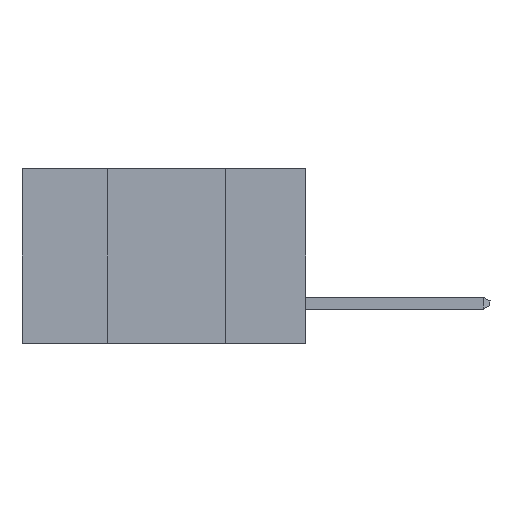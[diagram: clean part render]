
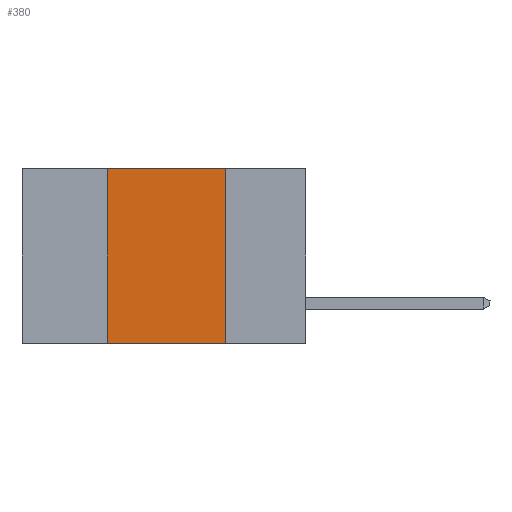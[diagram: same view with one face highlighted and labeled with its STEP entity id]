
A CAD part, left-side view. The second image highlights one B-rep face of the part: STEP entity #380.
In plain terms, the highlighted planar face has unit normal (-1, 0, 0).
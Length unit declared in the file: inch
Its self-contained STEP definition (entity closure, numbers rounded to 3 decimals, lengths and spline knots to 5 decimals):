
#60 = EDGE_LOOP ( 'NONE', ( #5931, #14650, #10827, #14016 ) ) ;
#380 = ADVANCED_FACE ( 'NONE', ( #4554 ), #8325, .F. ) ;
#771 = EDGE_CURVE ( 'NONE', #11678, #6938, #6595, .T. ) ;
#1671 = DIRECTION ( 'NONE',  ( 0., -1., 0. ) ) ;
#2271 = DIRECTION ( 'NONE',  ( 0., -1., 0. ) ) ;
#2495 = EDGE_CURVE ( 'NONE', #8354, #11678, #5177, .T. ) ;
#2605 = CARTESIAN_POINT ( 'NONE',  ( 0., 0.6, 0. ) ) ;
#3304 = LINE ( 'NONE', #3466, #9718 ) ;
#3466 = CARTESIAN_POINT ( 'NONE',  ( 0., 0.42, -0.37 ) ) ;
#4554 = FACE_OUTER_BOUND ( 'NONE', #60, .T. ) ;
#5177 = LINE ( 'NONE', #2605, #11766 ) ;
#5626 = CARTESIAN_POINT ( 'NONE',  ( 0., 0.42, -0.37 ) ) ;
#5931 = ORIENTED_EDGE ( 'NONE', *, *, #771, .F. ) ;
#6094 = LINE ( 'NONE', #8217, #9256 ) ;
#6595 = LINE ( 'NONE', #10203, #14183 ) ;
#6938 = VERTEX_POINT ( 'NONE', #8489 ) ;
#8171 = DIRECTION ( 'NONE',  ( 0., 0., 1. ) ) ;
#8217 = CARTESIAN_POINT ( 'NONE',  ( 0., 0.6, -0.37 ) ) ;
#8325 = PLANE ( 'NONE',  #10686 ) ;
#8354 = VERTEX_POINT ( 'NONE', #15215 ) ;
#8489 = CARTESIAN_POINT ( 'NONE',  ( 0., 0.17, -0.37 ) ) ;
#9256 = VECTOR ( 'NONE', #2271, 39.37008 ) ;
#9366 = CARTESIAN_POINT ( 'NONE',  ( 0., 0.6, 0. ) ) ;
#9718 = VECTOR ( 'NONE', #8171, 39.37008 ) ;
#10203 = CARTESIAN_POINT ( 'NONE',  ( 0., 0.17, -0.37 ) ) ;
#10682 = DIRECTION ( 'NONE',  ( 0., 0., -1. ) ) ;
#10686 = AXIS2_PLACEMENT_3D ( 'NONE', #9366, #12861, #10682 ) ;
#10827 = ORIENTED_EDGE ( 'NONE', *, *, #11284, .F. ) ;
#11284 = EDGE_CURVE ( 'NONE', #11973, #8354, #3304, .T. ) ;
#11678 = VERTEX_POINT ( 'NONE', #14186 ) ;
#11766 = VECTOR ( 'NONE', #1671, 39.37008 ) ;
#11973 = VERTEX_POINT ( 'NONE', #5626 ) ;
#12861 = DIRECTION ( 'NONE',  ( 1., 0., 0. ) ) ;
#13787 = DIRECTION ( 'NONE',  ( 0., 0., -1. ) ) ;
#14016 = ORIENTED_EDGE ( 'NONE', *, *, #14677, .T. ) ;
#14183 = VECTOR ( 'NONE', #13787, 39.37008 ) ;
#14186 = CARTESIAN_POINT ( 'NONE',  ( 0., 0.17, 0. ) ) ;
#14650 = ORIENTED_EDGE ( 'NONE', *, *, #2495, .F. ) ;
#14677 = EDGE_CURVE ( 'NONE', #11973, #6938, #6094, .T. ) ;
#15215 = CARTESIAN_POINT ( 'NONE',  ( 0., 0.42, 0. ) ) ;
